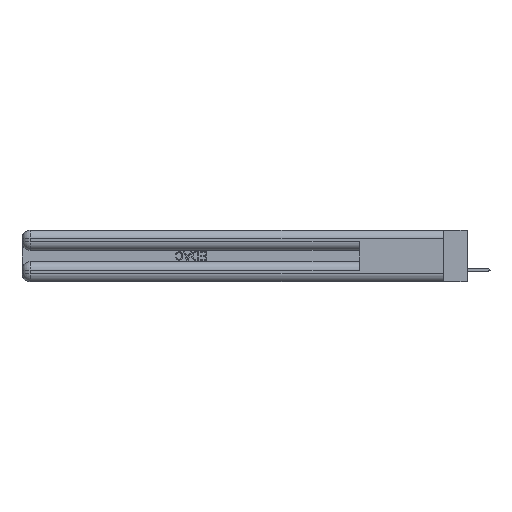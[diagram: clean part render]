
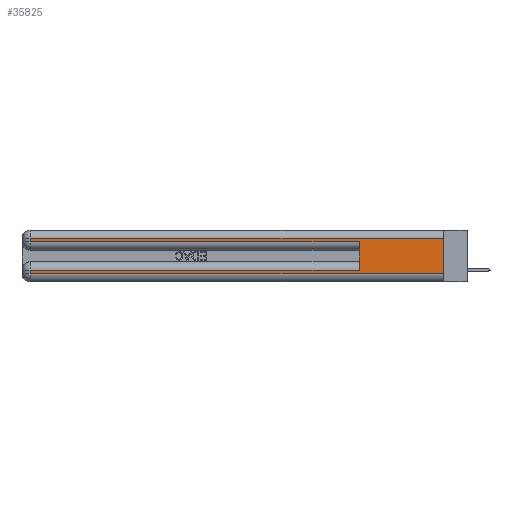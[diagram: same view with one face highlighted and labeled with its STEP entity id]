
A CAD part, left-side view. The second image highlights one B-rep face of the part: STEP entity #35825.
In plain terms, the highlighted planar face has unit normal (-1, 0, 0).
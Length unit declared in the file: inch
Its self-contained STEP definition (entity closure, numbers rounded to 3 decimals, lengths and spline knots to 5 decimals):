
#825 = ORIENTED_EDGE ( 'NONE', *, *, #16560, .F. ) ;
#977 = EDGE_CURVE ( 'NONE', #14023, #22300, #35197, .T. ) ;
#1432 = ORIENTED_EDGE ( 'NONE', *, *, #17118, .T. ) ;
#2043 = CARTESIAN_POINT ( 'NONE',  ( 0., 0.6, 0.145 ) ) ;
#4890 = DIRECTION ( 'NONE',  ( 0., 1., 0. ) ) ;
#5043 = VECTOR ( 'NONE', #48417, 39.37008 ) ;
#5529 = CARTESIAN_POINT ( 'NONE',  ( 0., 0., 0.37 ) ) ;
#6570 = LINE ( 'NONE', #29372, #13860 ) ;
#7551 = ORIENTED_EDGE ( 'NONE', *, *, #41774, .T. ) ;
#7800 = VERTEX_POINT ( 'NONE', #25012 ) ;
#8133 = EDGE_CURVE ( 'NONE', #11032, #7800, #54476, .T. ) ;
#8721 = LINE ( 'NONE', #2043, #26102 ) ;
#8979 = LINE ( 'NONE', #16842, #30380 ) ;
#9036 = ORIENTED_EDGE ( 'NONE', *, *, #8133, .T. ) ;
#11032 = VERTEX_POINT ( 'NONE', #27786 ) ;
#11154 = DIRECTION ( 'NONE',  ( 0., 1., 0. ) ) ;
#12201 = VECTOR ( 'NONE', #11154, 39.37008 ) ;
#12431 = CARTESIAN_POINT ( 'NONE',  ( 0., 0., 0.31 ) ) ;
#12846 = CARTESIAN_POINT ( 'NONE',  ( 0., 2.94, 0.37 ) ) ;
#13115 = ORIENTED_EDGE ( 'NONE', *, *, #23767, .T. ) ;
#13860 = VECTOR ( 'NONE', #38889, 39.37008 ) ;
#14023 = VERTEX_POINT ( 'NONE', #40882 ) ;
#15645 = CARTESIAN_POINT ( 'NONE',  ( 0., 0.6, 0.285 ) ) ;
#16259 = CARTESIAN_POINT ( 'NONE',  ( 0., 0., 0.37 ) ) ;
#16507 = VERTEX_POINT ( 'NONE', #12431 ) ;
#16560 = EDGE_CURVE ( 'NONE', #16507, #22300, #27818, .T. ) ;
#16842 = CARTESIAN_POINT ( 'NONE',  ( 0., 0., 0.285 ) ) ;
#16991 = VERTEX_POINT ( 'NONE', #25517 ) ;
#16997 = ORIENTED_EDGE ( 'NONE', *, *, #977, .T. ) ;
#17118 = EDGE_CURVE ( 'NONE', #36389, #34431, #8979, .T. ) ;
#17151 = DIRECTION ( 'NONE',  ( 1., 0., 0. ) ) ;
#19288 = ORIENTED_EDGE ( 'NONE', *, *, #45303, .T. ) ;
#21444 = DIRECTION ( 'NONE',  ( 0., 0., -1. ) ) ;
#22300 = VERTEX_POINT ( 'NONE', #45008 ) ;
#23767 = EDGE_CURVE ( 'NONE', #7800, #14023, #6570, .T. ) ;
#24454 = CARTESIAN_POINT ( 'NONE',  ( 0., 0., 0.085 ) ) ;
#25012 = CARTESIAN_POINT ( 'NONE',  ( 0., 2.94, 0.085 ) ) ;
#25234 = FACE_OUTER_BOUND ( 'NONE', #39940, .T. ) ;
#25312 = VECTOR ( 'NONE', #46972, 39.37008 ) ;
#25517 = CARTESIAN_POINT ( 'NONE',  ( 0., 2.94, 0.31 ) ) ;
#26102 = VECTOR ( 'NONE', #35742, 39.37008 ) ;
#26418 = CARTESIAN_POINT ( 'NONE',  ( 0., 0., 0.31 ) ) ;
#27386 = CARTESIAN_POINT ( 'NONE',  ( 0., 2.94, 0.285 ) ) ;
#27786 = CARTESIAN_POINT ( 'NONE',  ( 0., 0.6, 0.085 ) ) ;
#27818 = LINE ( 'NONE', #5529, #5043 ) ;
#28397 = DIRECTION ( 'NONE',  ( 0., -1., 0. ) ) ;
#28413 = EDGE_CURVE ( 'NONE', #11032, #34431, #8721, .T. ) ;
#29302 = LINE ( 'NONE', #12846, #25312 ) ;
#29372 = CARTESIAN_POINT ( 'NONE',  ( 0., 2.94, 0.37 ) ) ;
#30380 = VECTOR ( 'NONE', #28397, 39.37008 ) ;
#33911 = AXIS2_PLACEMENT_3D ( 'NONE', #16259, #17151, #21444 ) ;
#34431 = VERTEX_POINT ( 'NONE', #15645 ) ;
#35197 = LINE ( 'NONE', #39610, #35849 ) ;
#35742 = DIRECTION ( 'NONE',  ( 0., 0., 1. ) ) ;
#35825 = ADVANCED_FACE ( 'NONE', ( #25234 ), #54059, .F. ) ;
#35849 = VECTOR ( 'NONE', #53948, 39.37008 ) ;
#36389 = VERTEX_POINT ( 'NONE', #27386 ) ;
#38889 = DIRECTION ( 'NONE',  ( 0., 0., -1. ) ) ;
#38908 = VECTOR ( 'NONE', #4890, 39.37008 ) ;
#39610 = CARTESIAN_POINT ( 'NONE',  ( 0., 0., 0.06 ) ) ;
#39940 = EDGE_LOOP ( 'NONE', ( #825, #7551, #19288, #1432, #48001, #9036, #13115, #16997 ) ) ;
#40882 = CARTESIAN_POINT ( 'NONE',  ( 0., 2.94, 0.06 ) ) ;
#41774 = EDGE_CURVE ( 'NONE', #16507, #16991, #52988, .T. ) ;
#45008 = CARTESIAN_POINT ( 'NONE',  ( 0., 0., 0.06 ) ) ;
#45303 = EDGE_CURVE ( 'NONE', #16991, #36389, #29302, .T. ) ;
#46972 = DIRECTION ( 'NONE',  ( 0., 0., -1. ) ) ;
#48001 = ORIENTED_EDGE ( 'NONE', *, *, #28413, .F. ) ;
#48417 = DIRECTION ( 'NONE',  ( 0., 0., -1. ) ) ;
#52988 = LINE ( 'NONE', #26418, #38908 ) ;
#53948 = DIRECTION ( 'NONE',  ( 0., -1., 0. ) ) ;
#54059 = PLANE ( 'NONE',  #33911 ) ;
#54476 = LINE ( 'NONE', #24454, #12201 ) ;
